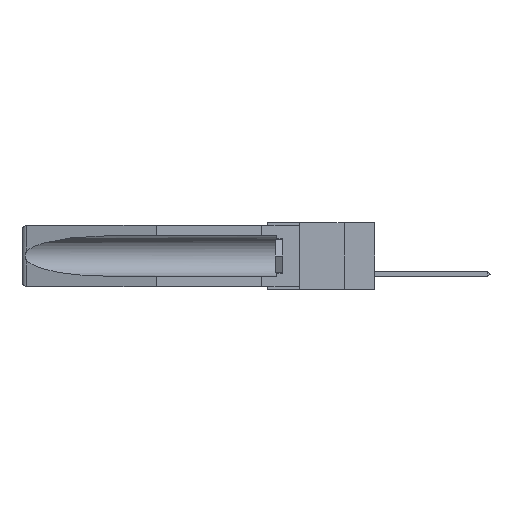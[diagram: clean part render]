
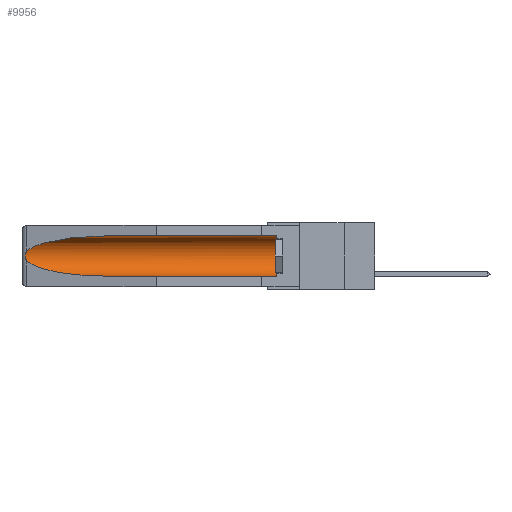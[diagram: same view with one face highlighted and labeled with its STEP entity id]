
A CAD part, left-side view. The second image highlights one B-rep face of the part: STEP entity #9956.
In plain terms, the highlighted cylindrical face has radius 2.857 mm (diameter 5.715 mm), a partial arc.
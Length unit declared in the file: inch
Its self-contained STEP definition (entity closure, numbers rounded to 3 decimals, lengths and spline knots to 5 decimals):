
#840 = CARTESIAN_POINT ( 'NONE',  ( 0.2673, 1.5327, -0.16383 ) ) ;
#1531 = CARTESIAN_POINT ( 'NONE',  ( 0.26537, 1.52718, -0.19328 ) ) ;
#2445 = VERTEX_POINT ( 'NONE', #10829 ) ;
#2671 = EDGE_CURVE ( 'NONE', #2445, #16597, #9626, .T. ) ;
#2819 = DIRECTION ( 'NONE',  ( 0., 0., 1. ) ) ;
#3140 = CARTESIAN_POINT ( 'NONE',  ( 0.155, -0.30754, -0.059 ) ) ;
#3213 = DIRECTION ( 'NONE',  ( 0., -1., 0. ) ) ;
#3925 = EDGE_CURVE ( 'NONE', #28284, #7379, #12763, .T. ) ;
#4129 = CARTESIAN_POINT ( 'NONE',  ( 0.155, -0.30754, -0.284 ) ) ;
#4160 = CARTESIAN_POINT ( 'NONE',  ( 0.21114, 1.30732, -0.059 ) ) ;
#4273 = CARTESIAN_POINT ( 'NONE',  ( 0.25451, 1.48313, -0.24835 ) ) ;
#4616 = EDGE_CURVE ( 'NONE', #7379, #22992, #18629, .T. ) ;
#5364 = DIRECTION ( 'NONE',  ( 0., 1., 0. ) ) ;
#5707 = VECTOR ( 'NONE', #26181, 39.37008 ) ;
#6084 = AXIS2_PLACEMENT_3D ( 'NONE', #15816, #16205, #27150 ) ;
#6296 = CARTESIAN_POINT ( 'NONE',  ( 0.155, 1.07973, -0.059 ) ) ;
#6667 = CARTESIAN_POINT ( 'NONE',  ( 0.26537, 1.52718, -0.14972 ) ) ;
#7062 = EDGE_CURVE ( 'NONE', #20516, #28284, #9146, .T. ) ;
#7148 = CARTESIAN_POINT ( 'NONE',  ( 0.2675, 1.53308, -0.16763 ) ) ;
#7379 = VERTEX_POINT ( 'NONE', #1531 ) ;
#8869 = CARTESIAN_POINT ( 'NONE',  ( 0.21114, 1.30732, -0.284 ) ) ;
#9146 =( BOUNDED_CURVE ( )  B_SPLINE_CURVE ( 3, ( #6296, #4160, #24154, #6667 ),
 .UNSPECIFIED., .F., .F. ) 
 B_SPLINE_CURVE_WITH_KNOTS ( ( 4, 4 ),
 ( 4.71239, 6.08839 ),
 .UNSPECIFIED. ) 
 CURVE ( )  GEOMETRIC_REPRESENTATION_ITEM ( )  RATIONAL_B_SPLINE_CURVE ( ( 1., 0.848, 0.848, 1. ) ) 
 REPRESENTATION_ITEM ( '' )  );
#9407 = ORIENTED_EDGE ( 'NONE', *, *, #7062, .T. ) ;
#9626 = CIRCLE ( 'NONE', #20740, 0.1125 ) ;
#9627 = ORIENTED_EDGE ( 'NONE', *, *, #24963, .T. ) ;
#9747 = CARTESIAN_POINT ( 'NONE',  ( 0.155, 0.126, -0.1715 ) ) ;
#9956 = ADVANCED_FACE ( 'NONE', ( #25037 ), #19443, .F. ) ;
#10829 = CARTESIAN_POINT ( 'NONE',  ( 0.155, 0.126, -0.284 ) ) ;
#11269 = EDGE_CURVE ( 'NONE', #2445, #22992, #23500, .T. ) ;
#11757 = CARTESIAN_POINT ( 'NONE',  ( 0.26597, 1.5296, -0.19026 ) ) ;
#11850 = CARTESIAN_POINT ( 'NONE',  ( 0.26597, 1.52961, -0.15275 ) ) ;
#12763 = B_SPLINE_CURVE_WITH_KNOTS ( 'NONE', 3,
 ( #14183, #11850, #27559, #840, #7148, #16134, #25310, #16428, #11757, #22756 ),
 .UNSPECIFIED., .F., .F.,
 ( 4, 2, 2, 2, 4 ),
 ( 0., 0.00029, 0.00058, 0.00087, 0.00117 ),
 .UNSPECIFIED. ) ;
#12884 = VECTOR ( 'NONE', #5364, 39.37008 ) ;
#13202 = CARTESIAN_POINT ( 'NONE',  ( 0.26537, 1.52718, -0.14972 ) ) ;
#13281 = EDGE_LOOP ( 'NONE', ( #9407, #23216, #20116, #22534, #19333, #9627 ) ) ;
#14183 = CARTESIAN_POINT ( 'NONE',  ( 0.26537, 1.52718, -0.14972 ) ) ;
#15816 = CARTESIAN_POINT ( 'NONE',  ( 0.155, -0.30754, -0.1715 ) ) ;
#16134 = CARTESIAN_POINT ( 'NONE',  ( 0.2675, 1.53308, -0.17534 ) ) ;
#16205 = DIRECTION ( 'NONE',  ( 0., 1., 0. ) ) ;
#16428 = CARTESIAN_POINT ( 'NONE',  ( 0.26655, 1.53094, -0.18657 ) ) ;
#16597 = VERTEX_POINT ( 'NONE', #17368 ) ;
#17368 = CARTESIAN_POINT ( 'NONE',  ( 0.155, 0.126, -0.059 ) ) ;
#17934 = CARTESIAN_POINT ( 'NONE',  ( 0.26537, 1.52718, -0.19328 ) ) ;
#18510 = CARTESIAN_POINT ( 'NONE',  ( 0.155, 1.07973, -0.284 ) ) ;
#18629 =( BOUNDED_CURVE ( )  B_SPLINE_CURVE ( 3, ( #17934, #4273, #8869, #20055 ),
 .UNSPECIFIED., .F., .F. ) 
 B_SPLINE_CURVE_WITH_KNOTS ( ( 4, 4 ),
 ( 0.1948, 1.5708 ),
 .UNSPECIFIED. ) 
 CURVE ( )  GEOMETRIC_REPRESENTATION_ITEM ( )  RATIONAL_B_SPLINE_CURVE ( ( 1., 0.848, 0.848, 1. ) ) 
 REPRESENTATION_ITEM ( '' )  );
#19333 = ORIENTED_EDGE ( 'NONE', *, *, #2671, .T. ) ;
#19443 = CYLINDRICAL_SURFACE ( 'NONE', #6084, 0.1125 ) ;
#20055 = CARTESIAN_POINT ( 'NONE',  ( 0.155, 1.07973, -0.284 ) ) ;
#20116 = ORIENTED_EDGE ( 'NONE', *, *, #4616, .T. ) ;
#20516 = VERTEX_POINT ( 'NONE', #27754 ) ;
#20740 = AXIS2_PLACEMENT_3D ( 'NONE', #9747, #3213, #2819 ) ;
#22301 = LINE ( 'NONE', #3140, #12884 ) ;
#22534 = ORIENTED_EDGE ( 'NONE', *, *, #11269, .F. ) ;
#22756 = CARTESIAN_POINT ( 'NONE',  ( 0.26537, 1.52718, -0.19328 ) ) ;
#22992 = VERTEX_POINT ( 'NONE', #18510 ) ;
#23216 = ORIENTED_EDGE ( 'NONE', *, *, #3925, .T. ) ;
#23500 = LINE ( 'NONE', #4129, #5707 ) ;
#24154 = CARTESIAN_POINT ( 'NONE',  ( 0.25451, 1.48313, -0.09465 ) ) ;
#24963 = EDGE_CURVE ( 'NONE', #16597, #20516, #22301, .T. ) ;
#25037 = FACE_OUTER_BOUND ( 'NONE', #13281, .T. ) ;
#25310 = CARTESIAN_POINT ( 'NONE',  ( 0.2673, 1.53269, -0.17917 ) ) ;
#26181 = DIRECTION ( 'NONE',  ( 0., 1., 0. ) ) ;
#27150 = DIRECTION ( 'NONE',  ( 0., 0., 1. ) ) ;
#27559 = CARTESIAN_POINT ( 'NONE',  ( 0.26654, 1.53092, -0.15636 ) ) ;
#27754 = CARTESIAN_POINT ( 'NONE',  ( 0.155, 1.07973, -0.059 ) ) ;
#28284 = VERTEX_POINT ( 'NONE', #13202 ) ;
